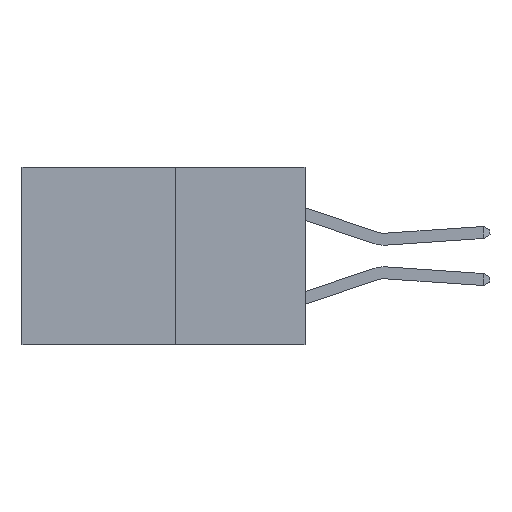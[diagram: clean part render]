
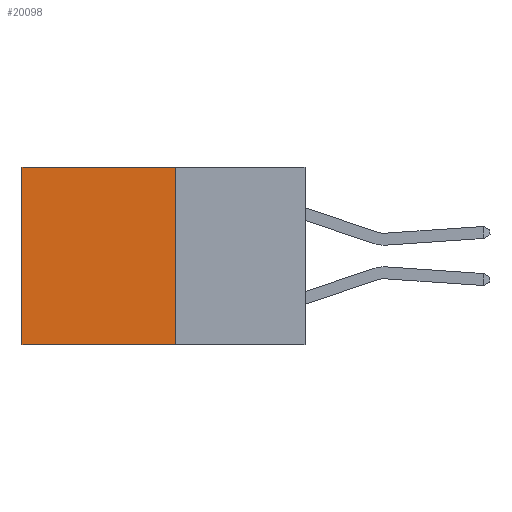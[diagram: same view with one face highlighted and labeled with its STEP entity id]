
A CAD part, left-side view. The second image highlights one B-rep face of the part: STEP entity #20098.
In plain terms, the highlighted planar face has unit normal (-1, 0, 0).
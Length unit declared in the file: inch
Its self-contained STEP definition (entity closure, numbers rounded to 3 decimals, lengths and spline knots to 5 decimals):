
#2707 = VERTEX_POINT ( 'NONE', #7950 ) ;
#4826 = CARTESIAN_POINT ( 'NONE',  ( 0.277, 0.27, -0.37 ) ) ;
#5198 = VERTEX_POINT ( 'NONE', #17942 ) ;
#5615 = LINE ( 'NONE', #14730, #19731 ) ;
#5898 = DIRECTION ( 'NONE',  ( 1., 0., 0. ) ) ;
#6146 = EDGE_CURVE ( 'NONE', #12806, #13743, #6609, .T. ) ;
#6258 = DIRECTION ( 'NONE',  ( 0., 0., -1. ) ) ;
#6609 = LINE ( 'NONE', #20696, #20697 ) ;
#7643 = CARTESIAN_POINT ( 'NONE',  ( 0.277, 0.59, 0. ) ) ;
#7950 = CARTESIAN_POINT ( 'NONE',  ( 0.277, 0.27, -0.37 ) ) ;
#8463 = ORIENTED_EDGE ( 'NONE', *, *, #9863, .F. ) ;
#8565 = ORIENTED_EDGE ( 'NONE', *, *, #19959, .T. ) ;
#8917 = VECTOR ( 'NONE', #6258, 39.37008 ) ;
#9863 = EDGE_CURVE ( 'NONE', #2707, #13743, #15199, .T. ) ;
#10354 = VECTOR ( 'NONE', #14165, 39.37008 ) ;
#11065 = DIRECTION ( 'NONE',  ( 0., 1., 0. ) ) ;
#12361 = FACE_OUTER_BOUND ( 'NONE', #21992, .T. ) ;
#12806 = VERTEX_POINT ( 'NONE', #7643 ) ;
#13275 = PLANE ( 'NONE',  #18074 ) ;
#13743 = VERTEX_POINT ( 'NONE', #22806 ) ;
#13826 = LINE ( 'NONE', #15448, #8917 ) ;
#14165 = DIRECTION ( 'NONE',  ( 0., 1., 0. ) ) ;
#14416 = EDGE_CURVE ( 'NONE', #5198, #2707, #13826, .T. ) ;
#14730 = CARTESIAN_POINT ( 'NONE',  ( 0.277, 0.27, 0. ) ) ;
#15199 = LINE ( 'NONE', #4826, #10354 ) ;
#15448 = CARTESIAN_POINT ( 'NONE',  ( 0.277, 0.27, -0.37 ) ) ;
#16941 = CARTESIAN_POINT ( 'NONE',  ( 0.277, 0.27, -0.37 ) ) ;
#17440 = ORIENTED_EDGE ( 'NONE', *, *, #14416, .F. ) ;
#17942 = CARTESIAN_POINT ( 'NONE',  ( 0.277, 0.27, 0. ) ) ;
#18074 = AXIS2_PLACEMENT_3D ( 'NONE', #16941, #5898, #18770 ) ;
#18770 = DIRECTION ( 'NONE',  ( 0., 0., -1. ) ) ;
#19731 = VECTOR ( 'NONE', #11065, 39.37008 ) ;
#19959 = EDGE_CURVE ( 'NONE', #5198, #12806, #5615, .T. ) ;
#20098 = ADVANCED_FACE ( 'NONE', ( #12361 ), #13275, .F. ) ;
#20368 = ORIENTED_EDGE ( 'NONE', *, *, #6146, .T. ) ;
#20696 = CARTESIAN_POINT ( 'NONE',  ( 0.277, 0.59, -0.37 ) ) ;
#20697 = VECTOR ( 'NONE', #21623, 39.37008 ) ;
#21623 = DIRECTION ( 'NONE',  ( 0., 0., -1. ) ) ;
#21992 = EDGE_LOOP ( 'NONE', ( #20368, #8463, #17440, #8565 ) ) ;
#22806 = CARTESIAN_POINT ( 'NONE',  ( 0.277, 0.59, -0.37 ) ) ;
